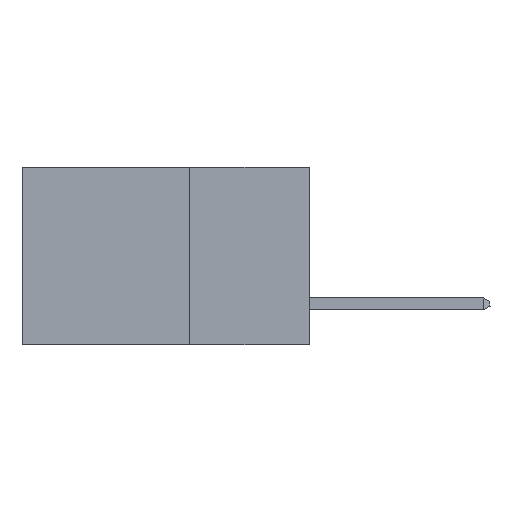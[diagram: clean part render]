
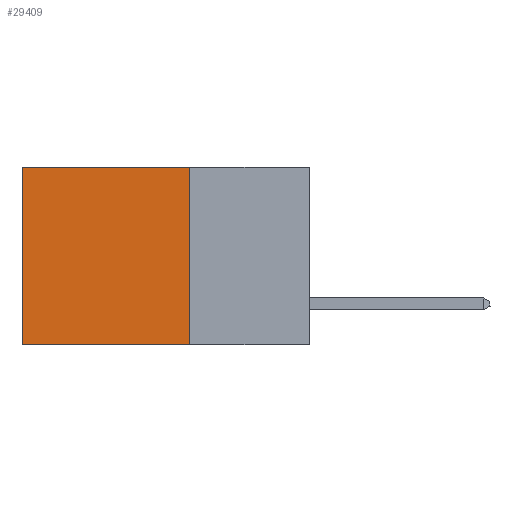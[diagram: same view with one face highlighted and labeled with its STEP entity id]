
A CAD part, left-side view. The second image highlights one B-rep face of the part: STEP entity #29409.
In plain terms, the highlighted planar face has unit normal (-1, 0, 0).
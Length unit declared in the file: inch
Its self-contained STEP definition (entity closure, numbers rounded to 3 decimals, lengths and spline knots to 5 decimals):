
#1462 = LINE ( 'NONE', #38673, #27454 ) ;
#1790 = ORIENTED_EDGE ( 'NONE', *, *, #28655, .F. ) ;
#3441 = PLANE ( 'NONE',  #26198 ) ;
#6210 = EDGE_CURVE ( 'NONE', #31122, #36979, #15675, .T. ) ;
#6758 = DIRECTION ( 'NONE',  ( 0., 0., -1. ) ) ;
#9547 = ORIENTED_EDGE ( 'NONE', *, *, #22677, .T. ) ;
#10271 = LINE ( 'NONE', #23646, #39399 ) ;
#11420 = VECTOR ( 'NONE', #11702, 39.37008 ) ;
#11546 = CARTESIAN_POINT ( 'NONE',  ( 0.2875, 0.25, -0.37 ) ) ;
#11702 = DIRECTION ( 'NONE',  ( 0., 1., 0. ) ) ;
#13652 = DIRECTION ( 'NONE',  ( 1., 0., 0. ) ) ;
#15675 = LINE ( 'NONE', #16411, #39580 ) ;
#16411 = CARTESIAN_POINT ( 'NONE',  ( 0.2875, 0.25, 0. ) ) ;
#20129 = ORIENTED_EDGE ( 'NONE', *, *, #6210, .F. ) ;
#20314 = CARTESIAN_POINT ( 'NONE',  ( 0.2875, 0.25, 0. ) ) ;
#20412 = LINE ( 'NONE', #11546, #11420 ) ;
#20749 = CARTESIAN_POINT ( 'NONE',  ( 0.2875, 0.25, 0. ) ) ;
#21751 = DIRECTION ( 'NONE',  ( 0., 1., 0. ) ) ;
#21901 = FACE_OUTER_BOUND ( 'NONE', #43008, .T. ) ;
#22032 = EDGE_CURVE ( 'NONE', #37613, #25696, #10271, .T. ) ;
#22677 = EDGE_CURVE ( 'NONE', #31122, #37613, #1462, .T. ) ;
#23646 = CARTESIAN_POINT ( 'NONE',  ( 0.2875, 0.6, 0. ) ) ;
#25696 = VERTEX_POINT ( 'NONE', #30794 ) ;
#26198 = AXIS2_PLACEMENT_3D ( 'NONE', #20749, #13652, #37354 ) ;
#27440 = CARTESIAN_POINT ( 'NONE',  ( 0.2875, 0.6, 0. ) ) ;
#27454 = VECTOR ( 'NONE', #21751, 39.37008 ) ;
#28655 = EDGE_CURVE ( 'NONE', #36979, #25696, #20412, .T. ) ;
#29409 = ADVANCED_FACE ( 'NONE', ( #21901 ), #3441, .F. ) ;
#30794 = CARTESIAN_POINT ( 'NONE',  ( 0.2875, 0.6, -0.37 ) ) ;
#31122 = VERTEX_POINT ( 'NONE', #20314 ) ;
#34905 = ORIENTED_EDGE ( 'NONE', *, *, #22032, .T. ) ;
#36979 = VERTEX_POINT ( 'NONE', #43684 ) ;
#37354 = DIRECTION ( 'NONE',  ( 0., 0., -1. ) ) ;
#37613 = VERTEX_POINT ( 'NONE', #27440 ) ;
#38073 = DIRECTION ( 'NONE',  ( 0., 0., -1. ) ) ;
#38673 = CARTESIAN_POINT ( 'NONE',  ( 0.2875, 0.25, 0. ) ) ;
#39399 = VECTOR ( 'NONE', #6758, 39.37008 ) ;
#39580 = VECTOR ( 'NONE', #38073, 39.37008 ) ;
#43008 = EDGE_LOOP ( 'NONE', ( #34905, #1790, #20129, #9547 ) ) ;
#43684 = CARTESIAN_POINT ( 'NONE',  ( 0.2875, 0.25, -0.37 ) ) ;
